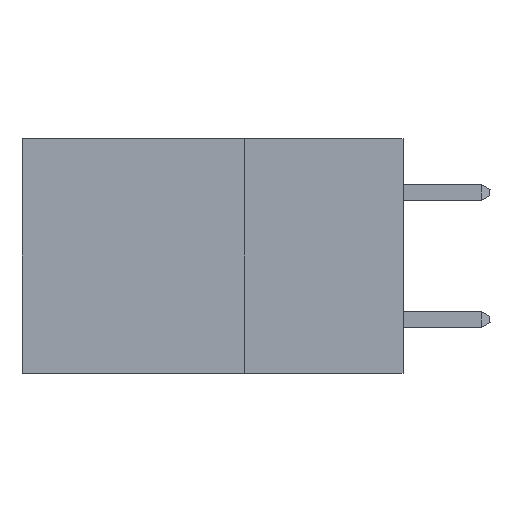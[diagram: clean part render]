
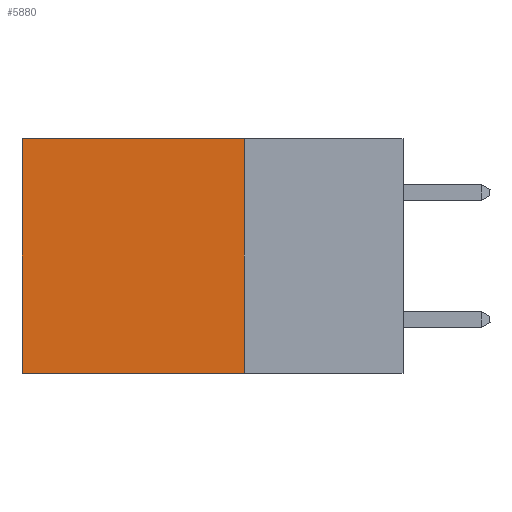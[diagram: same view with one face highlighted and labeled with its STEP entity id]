
A CAD part, left-side view. The second image highlights one B-rep face of the part: STEP entity #5880.
In plain terms, the highlighted planar face has unit normal (-1, 0, 0).
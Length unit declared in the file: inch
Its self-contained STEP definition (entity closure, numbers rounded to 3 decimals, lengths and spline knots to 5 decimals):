
#1359 = VECTOR ( 'NONE', #6094, 39.37008 ) ;
#2458 = DIRECTION ( 'NONE',  ( 0., 1., 0. ) ) ;
#3157 = EDGE_LOOP ( 'NONE', ( #5130, #16174, #18391, #21000 ) ) ;
#3264 = CARTESIAN_POINT ( 'NONE',  ( 0.2875, 0.6, 0. ) ) ;
#4043 = VERTEX_POINT ( 'NONE', #18896 ) ;
#4217 = LINE ( 'NONE', #15580, #20546 ) ;
#4247 = CARTESIAN_POINT ( 'NONE',  ( 0.2875, 0.25, 0. ) ) ;
#5130 = ORIENTED_EDGE ( 'NONE', *, *, #8934, .T. ) ;
#5880 = ADVANCED_FACE ( 'NONE', ( #17263 ), #15719, .F. ) ;
#6094 = DIRECTION ( 'NONE',  ( 0., 0., -1. ) ) ;
#6143 = CARTESIAN_POINT ( 'NONE',  ( 0.2875, 0.6, -0.37 ) ) ;
#6308 = DIRECTION ( 'NONE',  ( 0., 1., 0. ) ) ;
#7555 = DIRECTION ( 'NONE',  ( 0., 0., -1. ) ) ;
#8238 = EDGE_CURVE ( 'NONE', #4043, #11672, #4217, .T. ) ;
#8934 = EDGE_CURVE ( 'NONE', #11672, #16431, #18265, .T. ) ;
#9016 = EDGE_CURVE ( 'NONE', #14160, #16431, #12923, .T. ) ;
#11257 = DIRECTION ( 'NONE',  ( 0., 0., -1. ) ) ;
#11672 = VERTEX_POINT ( 'NONE', #3264 ) ;
#11723 = VECTOR ( 'NONE', #11257, 39.37008 ) ;
#12167 = AXIS2_PLACEMENT_3D ( 'NONE', #4247, #17358, #7555 ) ;
#12398 = VECTOR ( 'NONE', #6308, 39.37008 ) ;
#12923 = LINE ( 'NONE', #14488, #12398 ) ;
#14160 = VERTEX_POINT ( 'NONE', #21009 ) ;
#14488 = CARTESIAN_POINT ( 'NONE',  ( 0.2875, 0.25, -0.37 ) ) ;
#15580 = CARTESIAN_POINT ( 'NONE',  ( 0.2875, 0.25, 0. ) ) ;
#15719 = PLANE ( 'NONE',  #12167 ) ;
#16157 = CARTESIAN_POINT ( 'NONE',  ( 0.2875, 0.25, 0. ) ) ;
#16174 = ORIENTED_EDGE ( 'NONE', *, *, #9016, .F. ) ;
#16431 = VERTEX_POINT ( 'NONE', #6143 ) ;
#16522 = EDGE_CURVE ( 'NONE', #4043, #14160, #19851, .T. ) ;
#17263 = FACE_OUTER_BOUND ( 'NONE', #3157, .T. ) ;
#17358 = DIRECTION ( 'NONE',  ( 1., 0., 0. ) ) ;
#18265 = LINE ( 'NONE', #19148, #1359 ) ;
#18391 = ORIENTED_EDGE ( 'NONE', *, *, #16522, .F. ) ;
#18896 = CARTESIAN_POINT ( 'NONE',  ( 0.2875, 0.25, 0. ) ) ;
#19148 = CARTESIAN_POINT ( 'NONE',  ( 0.2875, 0.6, 0. ) ) ;
#19851 = LINE ( 'NONE', #16157, #11723 ) ;
#20546 = VECTOR ( 'NONE', #2458, 39.37008 ) ;
#21000 = ORIENTED_EDGE ( 'NONE', *, *, #8238, .T. ) ;
#21009 = CARTESIAN_POINT ( 'NONE',  ( 0.2875, 0.25, -0.37 ) ) ;
